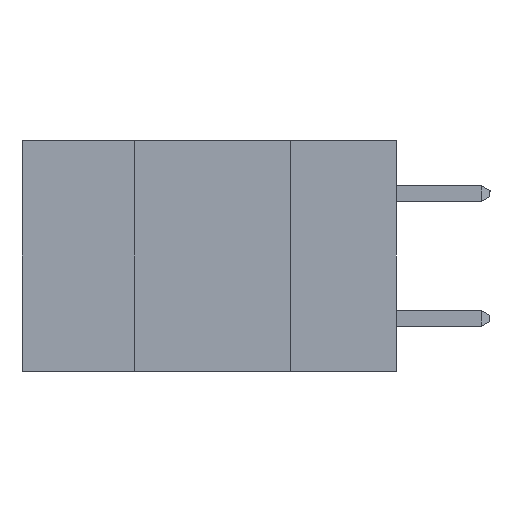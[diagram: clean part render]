
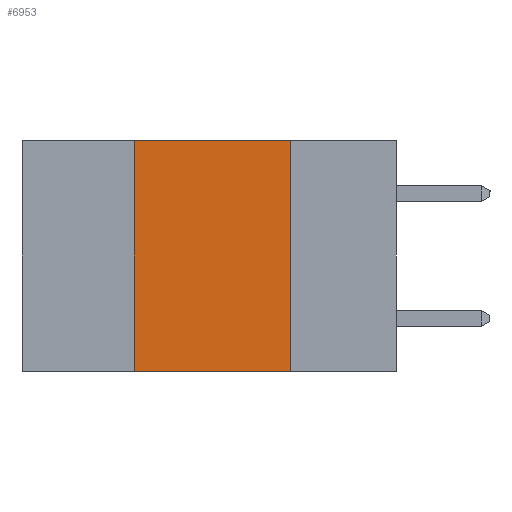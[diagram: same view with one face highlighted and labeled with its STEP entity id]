
A CAD part, left-side view. The second image highlights one B-rep face of the part: STEP entity #6953.
In plain terms, the highlighted planar face has unit normal (-1, 0, 0).
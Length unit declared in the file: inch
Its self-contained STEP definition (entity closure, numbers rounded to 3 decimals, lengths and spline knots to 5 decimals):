
#964 = DIRECTION ( 'NONE',  ( 0., -1., 0. ) ) ;
#974 = ORIENTED_EDGE ( 'NONE', *, *, #11165, .F. ) ;
#1726 = CARTESIAN_POINT ( 'NONE',  ( 0., 0.42, -0.37 ) ) ;
#1745 = VECTOR ( 'NONE', #10742, 39.37008 ) ;
#1942 = CARTESIAN_POINT ( 'NONE',  ( 0., 0.17, -0.37 ) ) ;
#2081 = EDGE_CURVE ( 'NONE', #10442, #6134, #12910, .T. ) ;
#2352 = ORIENTED_EDGE ( 'NONE', *, *, #2081, .F. ) ;
#2836 = LINE ( 'NONE', #12141, #13028 ) ;
#3032 = LINE ( 'NONE', #13226, #10733 ) ;
#3550 = AXIS2_PLACEMENT_3D ( 'NONE', #4975, #6006, #13175 ) ;
#4052 = EDGE_CURVE ( 'NONE', #10442, #7154, #3032, .T. ) ;
#4093 = DIRECTION ( 'NONE',  ( 0., -1., 0. ) ) ;
#4897 = CARTESIAN_POINT ( 'NONE',  ( 0., 0.17, 0. ) ) ;
#4975 = CARTESIAN_POINT ( 'NONE',  ( 0., 0.6, 0. ) ) ;
#6006 = DIRECTION ( 'NONE',  ( 1., 0., 0. ) ) ;
#6134 = VERTEX_POINT ( 'NONE', #13270 ) ;
#6616 = VECTOR ( 'NONE', #9135, 39.37008 ) ;
#6953 = ADVANCED_FACE ( 'NONE', ( #9050 ), #8025, .F. ) ;
#7154 = VERTEX_POINT ( 'NONE', #7409 ) ;
#7246 = EDGE_CURVE ( 'NONE', #6134, #7802, #2836, .T. ) ;
#7409 = CARTESIAN_POINT ( 'NONE',  ( 0., 0.17, -0.37 ) ) ;
#7802 = VERTEX_POINT ( 'NONE', #4897 ) ;
#8025 = PLANE ( 'NONE',  #3550 ) ;
#8880 = ORIENTED_EDGE ( 'NONE', *, *, #7246, .F. ) ;
#8917 = ORIENTED_EDGE ( 'NONE', *, *, #4052, .T. ) ;
#9050 = FACE_OUTER_BOUND ( 'NONE', #12162, .T. ) ;
#9135 = DIRECTION ( 'NONE',  ( 0., 0., -1. ) ) ;
#10442 = VERTEX_POINT ( 'NONE', #11263 ) ;
#10733 = VECTOR ( 'NONE', #4093, 39.37008 ) ;
#10742 = DIRECTION ( 'NONE',  ( 0., 0., 1. ) ) ;
#11165 = EDGE_CURVE ( 'NONE', #7802, #7154, #12883, .T. ) ;
#11263 = CARTESIAN_POINT ( 'NONE',  ( 0., 0.42, -0.37 ) ) ;
#12141 = CARTESIAN_POINT ( 'NONE',  ( 0., 0.6, 0. ) ) ;
#12162 = EDGE_LOOP ( 'NONE', ( #974, #8880, #2352, #8917 ) ) ;
#12883 = LINE ( 'NONE', #1942, #6616 ) ;
#12910 = LINE ( 'NONE', #1726, #1745 ) ;
#13028 = VECTOR ( 'NONE', #964, 39.37008 ) ;
#13175 = DIRECTION ( 'NONE',  ( 0., 0., -1. ) ) ;
#13226 = CARTESIAN_POINT ( 'NONE',  ( 0., 0.6, -0.37 ) ) ;
#13270 = CARTESIAN_POINT ( 'NONE',  ( 0., 0.42, 0. ) ) ;
